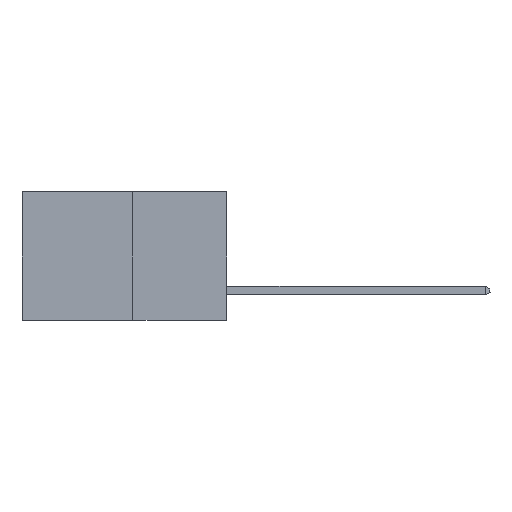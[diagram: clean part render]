
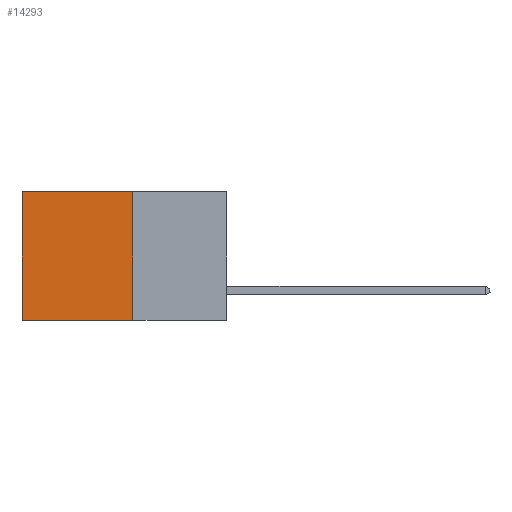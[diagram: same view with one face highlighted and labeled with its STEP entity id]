
A CAD part, left-side view. The second image highlights one B-rep face of the part: STEP entity #14293.
In plain terms, the highlighted planar face has unit normal (-1, 0, 0).
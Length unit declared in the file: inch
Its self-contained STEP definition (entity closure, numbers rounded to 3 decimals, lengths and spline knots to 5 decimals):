
#860 = EDGE_LOOP ( 'NONE', ( #16720, #19340, #17500, #7386 ) ) ;
#1141 = LINE ( 'NONE', #12030, #6044 ) ;
#2740 = EDGE_CURVE ( 'NONE', #11557, #15494, #7931, .T. ) ;
#3036 = CARTESIAN_POINT ( 'NONE',  ( 0.277, 0.59, 0. ) ) ;
#3732 = VECTOR ( 'NONE', #7436, 39.37008 ) ;
#5416 = DIRECTION ( 'NONE',  ( 0., 0., -1. ) ) ;
#6044 = VECTOR ( 'NONE', #13572, 39.37008 ) ;
#6175 = CARTESIAN_POINT ( 'NONE',  ( 0.277, 0.59, -0.37 ) ) ;
#6242 = CARTESIAN_POINT ( 'NONE',  ( 0.277, 0.27, -0.37 ) ) ;
#7000 = CARTESIAN_POINT ( 'NONE',  ( 0.277, 0.27, -0.37 ) ) ;
#7381 = AXIS2_PLACEMENT_3D ( 'NONE', #17708, #14742, #5416 ) ;
#7386 = ORIENTED_EDGE ( 'NONE', *, *, #14406, .T. ) ;
#7436 = DIRECTION ( 'NONE',  ( 0., 0., -1. ) ) ;
#7931 = LINE ( 'NONE', #6175, #3732 ) ;
#8536 = CARTESIAN_POINT ( 'NONE',  ( 0.277, 0.27, 0. ) ) ;
#9161 = LINE ( 'NONE', #6242, #12890 ) ;
#11557 = VERTEX_POINT ( 'NONE', #3036 ) ;
#11701 = PLANE ( 'NONE',  #7381 ) ;
#12030 = CARTESIAN_POINT ( 'NONE',  ( 0.277, 0.27, 0. ) ) ;
#12598 = VECTOR ( 'NONE', #19317, 39.37008 ) ;
#12890 = VECTOR ( 'NONE', #18596, 39.37008 ) ;
#13572 = DIRECTION ( 'NONE',  ( 0., 1., 0. ) ) ;
#13675 = VERTEX_POINT ( 'NONE', #8536 ) ;
#14293 = ADVANCED_FACE ( 'NONE', ( #19660 ), #11701, .F. ) ;
#14406 = EDGE_CURVE ( 'NONE', #13675, #11557, #1141, .T. ) ;
#14742 = DIRECTION ( 'NONE',  ( 1., 0., 0. ) ) ;
#15468 = CARTESIAN_POINT ( 'NONE',  ( 0.277, 0.27, -0.37 ) ) ;
#15494 = VERTEX_POINT ( 'NONE', #18201 ) ;
#16720 = ORIENTED_EDGE ( 'NONE', *, *, #2740, .T. ) ;
#17056 = LINE ( 'NONE', #7000, #12598 ) ;
#17500 = ORIENTED_EDGE ( 'NONE', *, *, #19386, .F. ) ;
#17627 = VERTEX_POINT ( 'NONE', #15468 ) ;
#17659 = EDGE_CURVE ( 'NONE', #17627, #15494, #9161, .T. ) ;
#17708 = CARTESIAN_POINT ( 'NONE',  ( 0.277, 0.27, -0.37 ) ) ;
#18201 = CARTESIAN_POINT ( 'NONE',  ( 0.277, 0.59, -0.37 ) ) ;
#18596 = DIRECTION ( 'NONE',  ( 0., 1., 0. ) ) ;
#19317 = DIRECTION ( 'NONE',  ( 0., 0., -1. ) ) ;
#19340 = ORIENTED_EDGE ( 'NONE', *, *, #17659, .F. ) ;
#19386 = EDGE_CURVE ( 'NONE', #13675, #17627, #17056, .T. ) ;
#19660 = FACE_OUTER_BOUND ( 'NONE', #860, .T. ) ;
